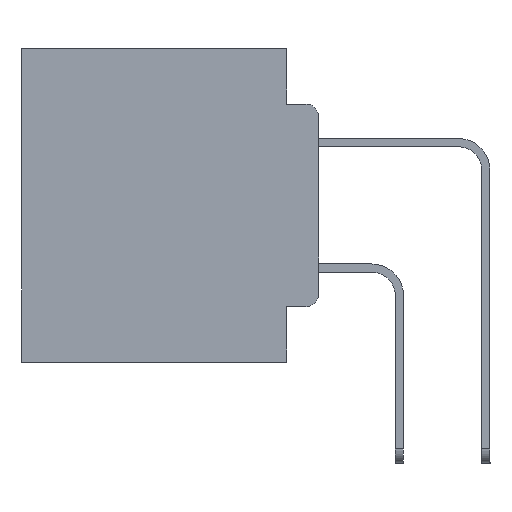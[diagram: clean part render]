
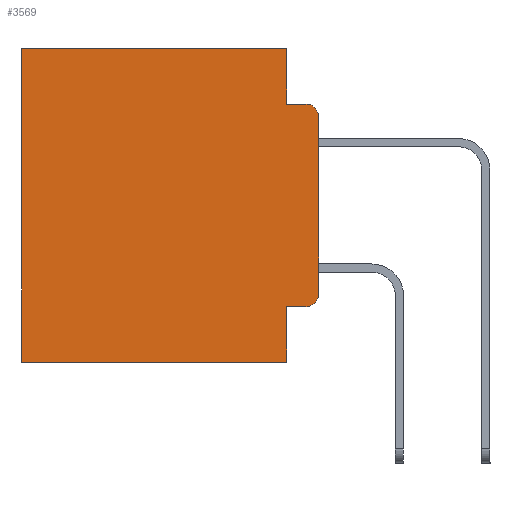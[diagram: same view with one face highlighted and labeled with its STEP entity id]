
A CAD part, left-side view. The second image highlights one B-rep face of the part: STEP entity #3569.
In plain terms, the highlighted planar face has unit normal (-1, 0, 0).
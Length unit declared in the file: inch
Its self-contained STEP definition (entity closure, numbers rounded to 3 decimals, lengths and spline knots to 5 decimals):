
#595 = ORIENTED_EDGE ( 'NONE', *, *, #12130, .F. ) ;
#1013 = DIRECTION ( 'NONE',  ( 0., 0., -1. ) ) ;
#2541 = VERTEX_POINT ( 'NONE', #22686 ) ;
#2846 = ORIENTED_EDGE ( 'NONE', *, *, #10271, .T. ) ;
#2882 = LINE ( 'NONE', #11601, #19418 ) ;
#2955 = CARTESIAN_POINT ( 'NONE',  ( 0.298, 0.051, -0.0885 ) ) ;
#3270 = VERTEX_POINT ( 'NONE', #18709 ) ;
#3569 = ADVANCED_FACE ( 'NONE', ( #25744 ), #15431, .F. ) ;
#4102 = DIRECTION ( 'NONE',  ( 0., -1., 0. ) ) ;
#4310 = DIRECTION ( 'NONE',  ( -1., 0., 0. ) ) ;
#4453 = EDGE_CURVE ( 'NONE', #2541, #6027, #10793, .T. ) ;
#4643 = AXIS2_PLACEMENT_3D ( 'NONE', #17214, #4310, #19326 ) ;
#4720 = CARTESIAN_POINT ( 'NONE',  ( 0.298, 0.473, -0.5 ) ) ;
#5253 = DIRECTION ( 'NONE',  ( 0., -1., 0. ) ) ;
#5514 = EDGE_CURVE ( 'NONE', #2541, #10758, #25193, .T. ) ;
#5581 = CARTESIAN_POINT ( 'NONE',  ( 0.298, 0., 0. ) ) ;
#5775 = VECTOR ( 'NONE', #15703, 39.37008 ) ;
#6027 = VERTEX_POINT ( 'NONE', #8020 ) ;
#6207 = VECTOR ( 'NONE', #4102, 39.37008 ) ;
#6379 = ORIENTED_EDGE ( 'NONE', *, *, #19988, .T. ) ;
#6574 = DIRECTION ( 'NONE',  ( 0., 0., -1. ) ) ;
#7583 = LINE ( 'NONE', #14933, #6207 ) ;
#8020 = CARTESIAN_POINT ( 'NONE',  ( 0.298, 0.473, 0. ) ) ;
#8323 = EDGE_CURVE ( 'NONE', #17387, #11072, #7583, .T. ) ;
#8346 = DIRECTION ( 'NONE',  ( -1., 0., 0. ) ) ;
#8436 = CARTESIAN_POINT ( 'NONE',  ( 0.298, 0.051, -0.4115 ) ) ;
#9327 = EDGE_CURVE ( 'NONE', #10758, #18539, #14903, .T. ) ;
#9551 = DIRECTION ( 'NONE',  ( 0., 1., 0. ) ) ;
#10030 = CIRCLE ( 'NONE', #4643, 0.02 ) ;
#10271 = EDGE_CURVE ( 'NONE', #3270, #18539, #22634, .T. ) ;
#10758 = VERTEX_POINT ( 'NONE', #22454 ) ;
#10793 = LINE ( 'NONE', #17024, #15792 ) ;
#11072 = VERTEX_POINT ( 'NONE', #19448 ) ;
#11601 = CARTESIAN_POINT ( 'NONE',  ( 0.298, 0.051, 0. ) ) ;
#11697 = EDGE_CURVE ( 'NONE', #11072, #25437, #10030, .T. ) ;
#12130 = EDGE_CURVE ( 'NONE', #3270, #25437, #16354, .T. ) ;
#12502 = DIRECTION ( 'NONE',  ( 0., 0., -1. ) ) ;
#12828 = ORIENTED_EDGE ( 'NONE', *, *, #8323, .T. ) ;
#12895 = DIRECTION ( 'NONE',  ( 1., 0., 0. ) ) ;
#13168 = AXIS2_PLACEMENT_3D ( 'NONE', #21049, #8346, #23099 ) ;
#13573 = CARTESIAN_POINT ( 'NONE',  ( 0.298, 0., -0.5 ) ) ;
#13759 = DIRECTION ( 'NONE',  ( 0., 0., -1. ) ) ;
#14127 = VECTOR ( 'NONE', #15170, 39.37008 ) ;
#14811 = ORIENTED_EDGE ( 'NONE', *, *, #5514, .F. ) ;
#14903 = LINE ( 'NONE', #2955, #25294 ) ;
#14933 = CARTESIAN_POINT ( 'NONE',  ( 0.298, 0.051, -0.4115 ) ) ;
#15120 = CARTESIAN_POINT ( 'NONE',  ( 0.298, 0., 0. ) ) ;
#15135 = CARTESIAN_POINT ( 'NONE',  ( 0.298, 0.051, 0. ) ) ;
#15170 = DIRECTION ( 'NONE',  ( 0., 0., -1. ) ) ;
#15431 = PLANE ( 'NONE',  #27005 ) ;
#15685 = VECTOR ( 'NONE', #1013, 39.37008 ) ;
#15703 = DIRECTION ( 'NONE',  ( 0., 1., 0. ) ) ;
#15792 = VECTOR ( 'NONE', #9551, 39.37008 ) ;
#15810 = EDGE_CURVE ( 'NONE', #18737, #18281, #27511, .T. ) ;
#16354 = LINE ( 'NONE', #5581, #15685 ) ;
#16688 = VECTOR ( 'NONE', #6574, 39.37008 ) ;
#17024 = CARTESIAN_POINT ( 'NONE',  ( 0.298, 0., 0. ) ) ;
#17214 = CARTESIAN_POINT ( 'NONE',  ( 0.298, 0.02, -0.3915 ) ) ;
#17342 = LINE ( 'NONE', #25470, #16688 ) ;
#17387 = VERTEX_POINT ( 'NONE', #8436 ) ;
#17437 = ORIENTED_EDGE ( 'NONE', *, *, #27497, .F. ) ;
#18281 = VERTEX_POINT ( 'NONE', #4720 ) ;
#18539 = VERTEX_POINT ( 'NONE', #18899 ) ;
#18709 = CARTESIAN_POINT ( 'NONE',  ( 0.298, 0., -0.1085 ) ) ;
#18737 = VERTEX_POINT ( 'NONE', #27784 ) ;
#18899 = CARTESIAN_POINT ( 'NONE',  ( 0.298, 0.02, -0.0885 ) ) ;
#19107 = CARTESIAN_POINT ( 'NONE',  ( 0.298, 0., -0.3915 ) ) ;
#19326 = DIRECTION ( 'NONE',  ( 0., 0., -1. ) ) ;
#19418 = VECTOR ( 'NONE', #13759, 39.37008 ) ;
#19448 = CARTESIAN_POINT ( 'NONE',  ( 0.298, 0.02, -0.4115 ) ) ;
#19988 = EDGE_CURVE ( 'NONE', #6027, #18281, #17342, .T. ) ;
#20699 = EDGE_LOOP ( 'NONE', ( #595, #2846, #26236, #14811, #22323, #6379, #24892, #17437, #12828, #25561 ) ) ;
#21049 = CARTESIAN_POINT ( 'NONE',  ( 0.298, 0.02, -0.1085 ) ) ;
#22323 = ORIENTED_EDGE ( 'NONE', *, *, #4453, .T. ) ;
#22454 = CARTESIAN_POINT ( 'NONE',  ( 0.298, 0.051, -0.0885 ) ) ;
#22634 = CIRCLE ( 'NONE', #13168, 0.02 ) ;
#22686 = CARTESIAN_POINT ( 'NONE',  ( 0.298, 0.051, 0. ) ) ;
#23099 = DIRECTION ( 'NONE',  ( 0., 0., -1. ) ) ;
#24892 = ORIENTED_EDGE ( 'NONE', *, *, #15810, .F. ) ;
#25193 = LINE ( 'NONE', #15135, #14127 ) ;
#25294 = VECTOR ( 'NONE', #5253, 39.37008 ) ;
#25437 = VERTEX_POINT ( 'NONE', #19107 ) ;
#25470 = CARTESIAN_POINT ( 'NONE',  ( 0.298, 0.473, 0. ) ) ;
#25561 = ORIENTED_EDGE ( 'NONE', *, *, #11697, .T. ) ;
#25744 = FACE_OUTER_BOUND ( 'NONE', #20699, .T. ) ;
#26236 = ORIENTED_EDGE ( 'NONE', *, *, #9327, .F. ) ;
#27005 = AXIS2_PLACEMENT_3D ( 'NONE', #15120, #12895, #12502 ) ;
#27497 = EDGE_CURVE ( 'NONE', #17387, #18737, #2882, .T. ) ;
#27511 = LINE ( 'NONE', #13573, #5775 ) ;
#27784 = CARTESIAN_POINT ( 'NONE',  ( 0.298, 0.051, -0.5 ) ) ;
